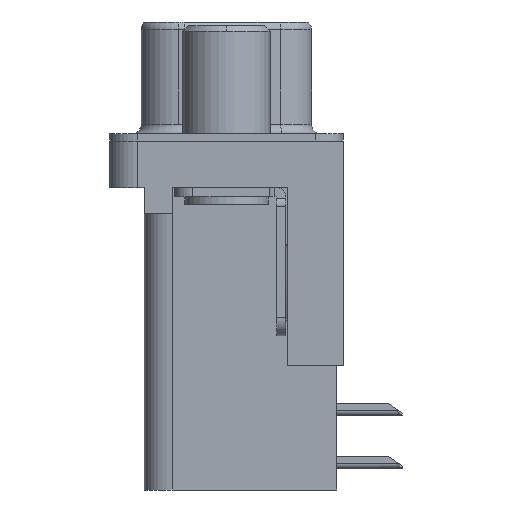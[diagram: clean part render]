
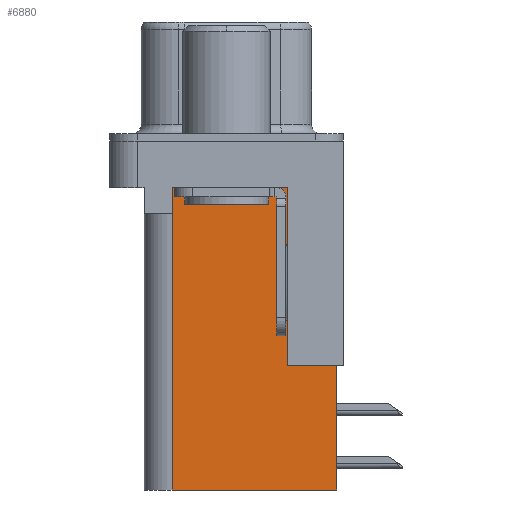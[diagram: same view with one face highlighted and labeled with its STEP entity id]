
A CAD part, left-side view. The second image highlights one B-rep face of the part: STEP entity #6880.
In plain terms, the highlighted planar face has unit normal (-1, 0, 0).
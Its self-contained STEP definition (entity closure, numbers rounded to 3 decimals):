
#161 = ORIENTED_EDGE ( 'NONE', *, *, #2246, .F. ) ;
#586 = DIRECTION ( 'NONE',  ( 0., 0., -1. ) ) ;
#675 = VECTOR ( 'NONE', #15211, 1000. ) ;
#818 = DIRECTION ( 'NONE',  ( 0., 1., 0. ) ) ;
#1326 = CARTESIAN_POINT ( 'NONE',  ( 3.765, 0., -3.9 ) ) ;
#1974 = EDGE_CURVE ( 'NONE', #8313, #18161, #3402, .T. ) ;
#1990 = LINE ( 'NONE', #9408, #18235 ) ;
#2089 = AXIS2_PLACEMENT_3D ( 'NONE', #18003, #7978, #5270 ) ;
#2246 = EDGE_CURVE ( 'NONE', #8837, #9665, #10701, .T. ) ;
#2319 = VECTOR ( 'NONE', #586, 1000. ) ;
#2430 = VECTOR ( 'NONE', #2908, 1000. ) ;
#2908 = DIRECTION ( 'NONE',  ( 0., 0., -1. ) ) ;
#3389 = ORIENTED_EDGE ( 'NONE', *, *, #17509, .T. ) ;
#3402 = LINE ( 'NONE', #15827, #15289 ) ;
#3481 = ORIENTED_EDGE ( 'NONE', *, *, #9591, .F. ) ;
#3917 = CARTESIAN_POINT ( 'NONE',  ( 3.765, -3.295, -18.76 ) ) ;
#4214 = CARTESIAN_POINT ( 'NONE',  ( 3.765, 2.895, -2.5 ) ) ;
#5270 = DIRECTION ( 'NONE',  ( 0., 1., 0. ) ) ;
#5661 = CARTESIAN_POINT ( 'NONE',  ( 3.765, -3.295, -2.5 ) ) ;
#5761 = ORIENTED_EDGE ( 'NONE', *, *, #1974, .T. ) ;
#5814 = VECTOR ( 'NONE', #7888, 1000. ) ;
#6387 = PLANE ( 'NONE',  #2089 ) ;
#6721 = LINE ( 'NONE', #20032, #2319 ) ;
#6880 = ADVANCED_FACE ( 'NONE', ( #20118 ), #6387, .F. ) ;
#7404 = VERTEX_POINT ( 'NONE', #15619 ) ;
#7843 = LINE ( 'NONE', #1326, #5814 ) ;
#7888 = DIRECTION ( 'NONE',  ( 0., 1., 0. ) ) ;
#7978 = DIRECTION ( 'NONE',  ( 1., 0., 0. ) ) ;
#8313 = VERTEX_POINT ( 'NONE', #17822 ) ;
#8674 = EDGE_LOOP ( 'NONE', ( #3389, #20217, #14729, #161, #14341, #3481, #5761, #8752 ) ) ;
#8752 = ORIENTED_EDGE ( 'NONE', *, *, #20849, .T. ) ;
#8837 = VERTEX_POINT ( 'NONE', #16208 ) ;
#9157 = DIRECTION ( 'NONE',  ( 0., 1., 0. ) ) ;
#9273 = CARTESIAN_POINT ( 'NONE',  ( 3.765, -3.295, -12.05 ) ) ;
#9408 = CARTESIAN_POINT ( 'NONE',  ( 3.765, -3.295, -18.76 ) ) ;
#9591 = EDGE_CURVE ( 'NONE', #8313, #16022, #14828, .T. ) ;
#9617 = EDGE_CURVE ( 'NONE', #14910, #9665, #7843, .T. ) ;
#9665 = VERTEX_POINT ( 'NONE', #15931 ) ;
#10701 = LINE ( 'NONE', #16661, #18853 ) ;
#12370 = CARTESIAN_POINT ( 'NONE',  ( 3.765, -5.925, -18.76 ) ) ;
#12544 = CARTESIAN_POINT ( 'NONE',  ( 3.765, -5.925, -2. ) ) ;
#12750 = EDGE_CURVE ( 'NONE', #16022, #8837, #1990, .T. ) ;
#13055 = LINE ( 'NONE', #3917, #675 ) ;
#13193 = VERTEX_POINT ( 'NONE', #4214 ) ;
#14153 = DIRECTION ( 'NONE',  ( 0., 1., 0. ) ) ;
#14341 = ORIENTED_EDGE ( 'NONE', *, *, #12750, .F. ) ;
#14729 = ORIENTED_EDGE ( 'NONE', *, *, #9617, .T. ) ;
#14828 = LINE ( 'NONE', #12544, #2430 ) ;
#14910 = VERTEX_POINT ( 'NONE', #15286 ) ;
#15159 = DIRECTION ( 'NONE',  ( 0., 0., 1. ) ) ;
#15211 = DIRECTION ( 'NONE',  ( 0., 0., 1. ) ) ;
#15286 = CARTESIAN_POINT ( 'NONE',  ( 3.765, 2.895, -3.9 ) ) ;
#15289 = VECTOR ( 'NONE', #9157, 1000. ) ;
#15489 = VECTOR ( 'NONE', #818, 1000. ) ;
#15619 = CARTESIAN_POINT ( 'NONE',  ( 3.765, -3.295, -2.5 ) ) ;
#15827 = CARTESIAN_POINT ( 'NONE',  ( 3.765, -6.295, -12.05 ) ) ;
#15931 = CARTESIAN_POINT ( 'NONE',  ( 3.765, 2.925, -3.9 ) ) ;
#16022 = VERTEX_POINT ( 'NONE', #12370 ) ;
#16208 = CARTESIAN_POINT ( 'NONE',  ( 3.765, 2.925, -18.76 ) ) ;
#16661 = CARTESIAN_POINT ( 'NONE',  ( 3.765, 2.925, -18.76 ) ) ;
#17509 = EDGE_CURVE ( 'NONE', #7404, #13193, #19834, .T. ) ;
#17822 = CARTESIAN_POINT ( 'NONE',  ( 3.765, -5.925, -12.05 ) ) ;
#17909 = EDGE_CURVE ( 'NONE', #13193, #14910, #6721, .T. ) ;
#18003 = CARTESIAN_POINT ( 'NONE',  ( 3.765, -3.295, -18.76 ) ) ;
#18161 = VERTEX_POINT ( 'NONE', #9273 ) ;
#18235 = VECTOR ( 'NONE', #14153, 1000. ) ;
#18853 = VECTOR ( 'NONE', #15159, 1000. ) ;
#19834 = LINE ( 'NONE', #5661, #15489 ) ;
#20032 = CARTESIAN_POINT ( 'NONE',  ( 3.765, 2.895, -3.9 ) ) ;
#20118 = FACE_OUTER_BOUND ( 'NONE', #8674, .T. ) ;
#20217 = ORIENTED_EDGE ( 'NONE', *, *, #17909, .T. ) ;
#20849 = EDGE_CURVE ( 'NONE', #18161, #7404, #13055, .T. ) ;
